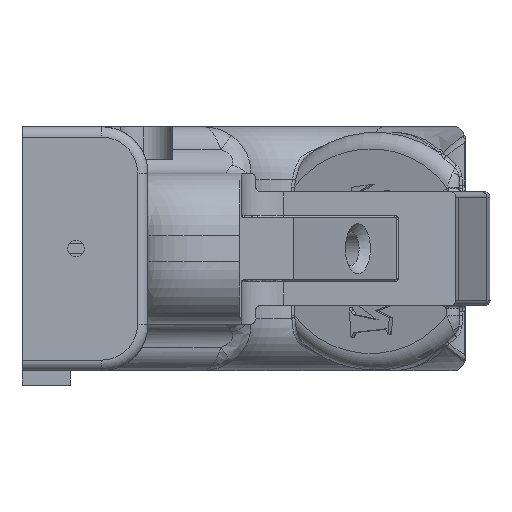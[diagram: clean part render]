
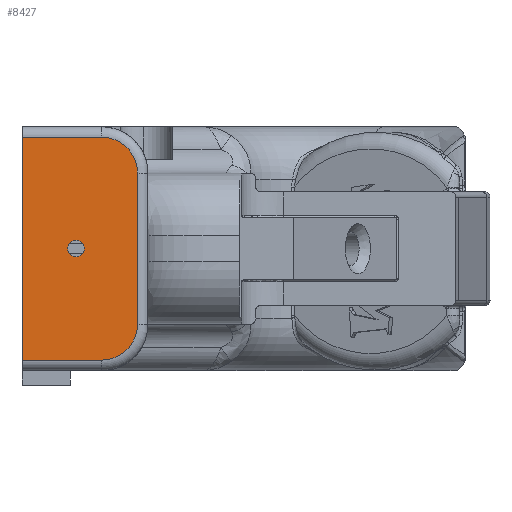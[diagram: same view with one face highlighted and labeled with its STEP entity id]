
A CAD part, left-side view. The second image highlights one B-rep face of the part: STEP entity #8427.
In plain terms, the highlighted planar face has unit normal (-1, 0, 0).
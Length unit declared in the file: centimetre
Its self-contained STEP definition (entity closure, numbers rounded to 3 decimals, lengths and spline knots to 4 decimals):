
#711=LINE($,#21658,#1400);
#915=LINE($,#22954,#1604);
#916=LINE($,#22956,#1605);
#917=LINE($,#22957,#1606);
#1400=VECTOR($,#10623,2.3019);
#1604=VECTOR($,#11237,1.212);
#1605=VECTOR($,#11238,3.3958);
#1606=VECTOR($,#11239,1.212);
#1937=PLANE($,#9192);
#2020=FACE_BOUND($,#2957,.T.);
#2437=FACE_OUTER_BOUND($,#2956,.T.);
#2956=EDGE_LOOP($,(#7339,#7340,#7341,#7342,#7343,#7344));
#2957=EDGE_LOOP($,(#7345));
#3264=CIRCLE($,#8985,0.125);
#3267=CIRCLE($,#8990,0.547);
#3271=CIRCLE($,#9008,0.547);
#3847=VERTEX_POINT($,#21652);
#3848=VERTEX_POINT($,#21655);
#3849=VERTEX_POINT($,#21657);
#3850=VERTEX_POINT($,#21661);
#3873=VERTEX_POINT($,#21723);
#4054=VERTEX_POINT($,#22953);
#4055=VERTEX_POINT($,#22955);
#4894=EDGE_CURVE($,#3847,#3847,#3264,.T.);
#4896=EDGE_CURVE($,#3848,#3849,#711,.T.);
#4898=EDGE_CURVE($,#3849,#3850,#3267,.T.);
#4928=EDGE_CURVE($,#3873,#3848,#3271,.T.);
#5217=EDGE_CURVE($,#4054,#3873,#915,.T.);
#5218=EDGE_CURVE($,#4054,#4055,#916,.T.);
#5219=EDGE_CURVE($,#3850,#4055,#917,.T.);
#7339=ORIENTED_EDGE($,*,*,#5217,.F.);
#7340=ORIENTED_EDGE($,*,*,#5218,.T.);
#7341=ORIENTED_EDGE($,*,*,#5219,.F.);
#7342=ORIENTED_EDGE($,*,*,#4898,.F.);
#7343=ORIENTED_EDGE($,*,*,#4896,.F.);
#7344=ORIENTED_EDGE($,*,*,#4928,.F.);
#7345=ORIENTED_EDGE($,*,*,#4894,.T.);
#8427=ADVANCED_FACE($,(#2437,#2020),#1937,.T.);
#8985=AXIS2_PLACEMENT_3D($,#21653,#10617,#10618);
#8990=AXIS2_PLACEMENT_3D($,#21662,#10628,#10629);
#9008=AXIS2_PLACEMENT_3D($,#21725,#10686,#10687);
#9192=AXIS2_PLACEMENT_3D($,#22952,#11235,#11236);
#10617=DIRECTION('center_axis',(1.,0.,0.));
#10618=DIRECTION('ref_axis',(0.,0.,
-1.));
#10623=DIRECTION($,(0.,0.,-1.));
#10628=DIRECTION('center_axis',(1.,0.,0.));
#10629=DIRECTION('ref_axis',(0.,-0.707,
-0.707));
#10686=DIRECTION('center_axis',(1.,0.,0.));
#10687=DIRECTION('ref_axis',(0.,-0.707,0.707));
#11235=DIRECTION('center_axis',(-1.,0.,0.));
#11236=DIRECTION('ref_axis',(0.,0.,1.));
#11237=DIRECTION($,(0.,-1.,0.));
#11238=DIRECTION($,(0.,0.,-1.));
#11239=DIRECTION($,(0.,1.,0.));
#21652=CARTESIAN_POINT('',(-19.1173,-0.2633,0.125));
#21653=CARTESIAN_POINT('Origin',(-19.1173,-0.2633,0.));
#21655=CARTESIAN_POINT('',(-19.1173,-1.2004,1.1509));
#21657=CARTESIAN_POINT('',(-19.1173,-1.2004,-1.1509));
#21658=CARTESIAN_POINT($,(-19.1173,-1.2004,-1.1509));
#21661=CARTESIAN_POINT('',(-19.1173,-0.6534,-1.6979));
#21662=CARTESIAN_POINT('Origin',(-19.1173,-0.6534,-1.1509));
#21723=CARTESIAN_POINT('',(-19.1173,-0.6534,1.6979));
#21725=CARTESIAN_POINT('Origin',(-19.1173,-0.6534,1.1509));
#22952=CARTESIAN_POINT('Origin',(-19.1173,-0.0777,
-1.1509));
#22953=CARTESIAN_POINT('',(-19.1173,0.5586,1.6979));
#22954=CARTESIAN_POINT($,(-19.1173,0.2405,1.6979));
#22955=CARTESIAN_POINT('',(-19.1173,0.5586,-1.6979));
#22956=CARTESIAN_POINT($,(-19.1173,0.5586,-1.7583));
#22957=CARTESIAN_POINT($,(-19.1173,0.2405,-1.6979));
